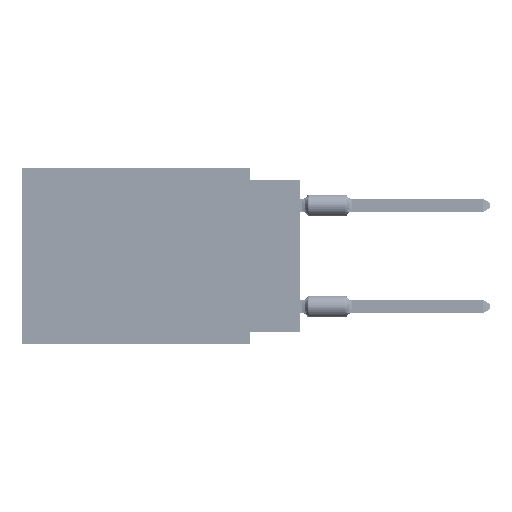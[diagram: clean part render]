
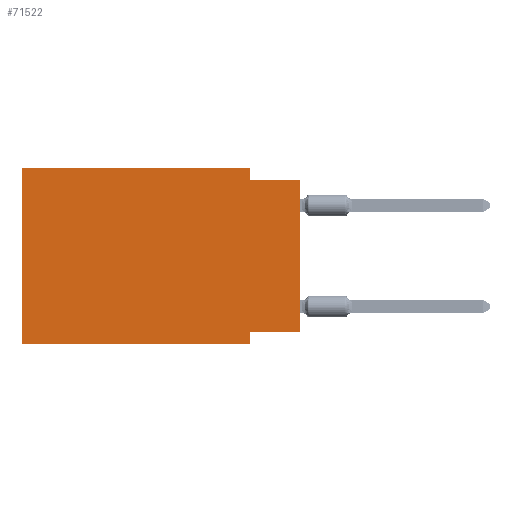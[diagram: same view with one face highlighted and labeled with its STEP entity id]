
A CAD part, left-side view. The second image highlights one B-rep face of the part: STEP entity #71522.
In plain terms, the highlighted planar face has unit normal (-1, 0, 0).
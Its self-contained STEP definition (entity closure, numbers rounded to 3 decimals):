
#519 = CARTESIAN_POINT ( 'NONE',  ( 0., 0., -0.635 ) ) ;
#1256 = CARTESIAN_POINT ( 'NONE',  ( 0., 2.54, 0. ) ) ;
#2162 = EDGE_CURVE ( 'NONE', #66093, #5060, #19991, .T. ) ;
#2974 = EDGE_CURVE ( 'NONE', #26205, #11414, #87979, .T. ) ;
#5060 = VERTEX_POINT ( 'NONE', #519 ) ;
#8624 = DIRECTION ( 'NONE',  ( 0., 0., -1. ) ) ;
#9310 = ORIENTED_EDGE ( 'NONE', *, *, #69689, .F. ) ;
#9689 = CARTESIAN_POINT ( 'NONE',  ( 0., 2.54, -8.255 ) ) ;
#10522 = ORIENTED_EDGE ( 'NONE', *, *, #50446, .F. ) ;
#11414 = VERTEX_POINT ( 'NONE', #95737 ) ;
#13025 = VERTEX_POINT ( 'NONE', #44702 ) ;
#14298 = CARTESIAN_POINT ( 'NONE',  ( 0., 13.97, 0. ) ) ;
#15287 = VECTOR ( 'NONE', #75150, 1000. ) ;
#15299 = CARTESIAN_POINT ( 'NONE',  ( 0., 2.54, -0.635 ) ) ;
#16180 = CARTESIAN_POINT ( 'NONE',  ( 0., 13.97, 0. ) ) ;
#17307 = VECTOR ( 'NONE', #54756, 1000. ) ;
#19991 = LINE ( 'NONE', #44265, #15287 ) ;
#21247 = CARTESIAN_POINT ( 'NONE',  ( 0., 2.54, 0. ) ) ;
#21760 = CARTESIAN_POINT ( 'NONE',  ( 0., 2.54, -8.89 ) ) ;
#24653 = DIRECTION ( 'NONE',  ( 0., 0., 1. ) ) ;
#25826 = VECTOR ( 'NONE', #24653, 1000. ) ;
#26205 = VERTEX_POINT ( 'NONE', #97546 ) ;
#28853 = VERTEX_POINT ( 'NONE', #21247 ) ;
#29415 = CARTESIAN_POINT ( 'NONE',  ( 0., 13.97, 0. ) ) ;
#31775 = EDGE_CURVE ( 'NONE', #13025, #78609, #84981, .T. ) ;
#32133 = DIRECTION ( 'NONE',  ( 0., 0., -1. ) ) ;
#37498 = DIRECTION ( 'NONE',  ( 0., -1., 0. ) ) ;
#44265 = CARTESIAN_POINT ( 'NONE',  ( 0., 0., -0.635 ) ) ;
#44702 = CARTESIAN_POINT ( 'NONE',  ( 0., 0., -8.255 ) ) ;
#45792 = ORIENTED_EDGE ( 'NONE', *, *, #93184, .F. ) ;
#46037 = VECTOR ( 'NONE', #46481, 1000. ) ;
#46232 = VERTEX_POINT ( 'NONE', #16180 ) ;
#46383 = ORIENTED_EDGE ( 'NONE', *, *, #96394, .T. ) ;
#46481 = DIRECTION ( 'NONE',  ( 0., 1., 0. ) ) ;
#47920 = LINE ( 'NONE', #78322, #25826 ) ;
#48127 = ORIENTED_EDGE ( 'NONE', *, *, #2974, .T. ) ;
#50248 = VECTOR ( 'NONE', #37498, 1000. ) ;
#50446 = EDGE_CURVE ( 'NONE', #78609, #11414, #91125, .T. ) ;
#50804 = LINE ( 'NONE', #96370, #50248 ) ;
#54693 = PLANE ( 'NONE',  #56893 ) ;
#54756 = DIRECTION ( 'NONE',  ( 0., 0., 1. ) ) ;
#55089 = ORIENTED_EDGE ( 'NONE', *, *, #2162, .F. ) ;
#55903 = LINE ( 'NONE', #1256, #90483 ) ;
#56353 = CARTESIAN_POINT ( 'NONE',  ( 0., 0., -8.255 ) ) ;
#56893 = AXIS2_PLACEMENT_3D ( 'NONE', #29415, #77987, #8624 ) ;
#58895 = EDGE_CURVE ( 'NONE', #28853, #66093, #55903, .T. ) ;
#62981 = ORIENTED_EDGE ( 'NONE', *, *, #31775, .F. ) ;
#65690 = CARTESIAN_POINT ( 'NONE',  ( 0., 13.97, -8.89 ) ) ;
#66093 = VERTEX_POINT ( 'NONE', #15299 ) ;
#68344 = VECTOR ( 'NONE', #83539, 1000. ) ;
#69559 = ORIENTED_EDGE ( 'NONE', *, *, #58895, .F. ) ;
#69689 = EDGE_CURVE ( 'NONE', #46232, #28853, #50804, .T. ) ;
#71522 = ADVANCED_FACE ( 'NONE', ( #76995 ), #54693, .F. ) ;
#75150 = DIRECTION ( 'NONE',  ( 0., -1., 0. ) ) ;
#76063 = LINE ( 'NONE', #14298, #17307 ) ;
#76995 = FACE_OUTER_BOUND ( 'NONE', #78356, .T. ) ;
#77987 = DIRECTION ( 'NONE',  ( 1., 0., 0. ) ) ;
#78322 = CARTESIAN_POINT ( 'NONE',  ( 0., 0., 0. ) ) ;
#78356 = EDGE_LOOP ( 'NONE', ( #46383, #55089, #69559, #9310, #45792, #48127, #10522, #62981 ) ) ;
#78609 = VERTEX_POINT ( 'NONE', #9689 ) ;
#83217 = VECTOR ( 'NONE', #96557, 1000. ) ;
#83539 = DIRECTION ( 'NONE',  ( 0., 0., -1. ) ) ;
#84981 = LINE ( 'NONE', #56353, #46037 ) ;
#87979 = LINE ( 'NONE', #65690, #83217 ) ;
#90483 = VECTOR ( 'NONE', #32133, 1000. ) ;
#91125 = LINE ( 'NONE', #21760, #68344 ) ;
#93184 = EDGE_CURVE ( 'NONE', #26205, #46232, #76063, .T. ) ;
#95737 = CARTESIAN_POINT ( 'NONE',  ( 0., 2.54, -8.89 ) ) ;
#96370 = CARTESIAN_POINT ( 'NONE',  ( 0., 13.97, 0. ) ) ;
#96394 = EDGE_CURVE ( 'NONE', #13025, #5060, #47920, .T. ) ;
#96557 = DIRECTION ( 'NONE',  ( 0., -1., 0. ) ) ;
#97546 = CARTESIAN_POINT ( 'NONE',  ( 0., 13.97, -8.89 ) ) ;
